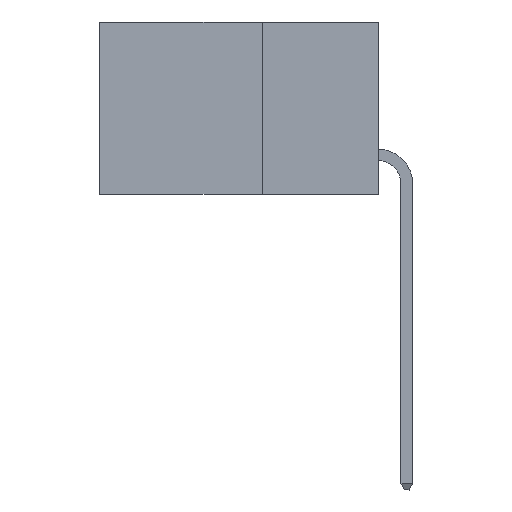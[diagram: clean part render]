
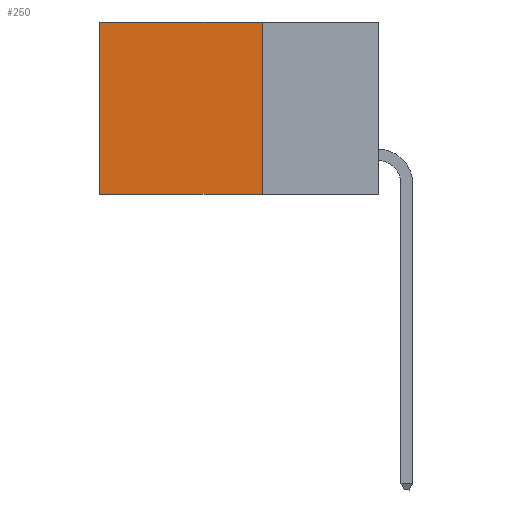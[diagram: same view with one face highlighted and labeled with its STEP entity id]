
A CAD part, left-side view. The second image highlights one B-rep face of the part: STEP entity #250.
In plain terms, the highlighted planar face has unit normal (-1, 0, 0).
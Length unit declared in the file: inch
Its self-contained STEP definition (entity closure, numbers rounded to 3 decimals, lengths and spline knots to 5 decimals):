
#130 = ORIENTED_EDGE ( 'NONE', *, *, #15612, .F. ) ;
#187 = CARTESIAN_POINT ( 'NONE',  ( 0.2615, 0.6, -0.37 ) ) ;
#250 = ADVANCED_FACE ( 'NONE', ( #16283 ), #5574, .F. ) ;
#1062 = LINE ( 'NONE', #5492, #11405 ) ;
#2078 = DIRECTION ( 'NONE',  ( 0., 0., -1. ) ) ;
#2416 = DIRECTION ( 'NONE',  ( 1., 0., 0. ) ) ;
#2471 = CARTESIAN_POINT ( 'NONE',  ( 0.2615, 0.25, -0.37 ) ) ;
#2823 = VECTOR ( 'NONE', #10074, 39.37008 ) ;
#4097 = AXIS2_PLACEMENT_3D ( 'NONE', #14981, #2416, #13232 ) ;
#4215 = DIRECTION ( 'NONE',  ( 0., 1., 0. ) ) ;
#4545 = EDGE_CURVE ( 'NONE', #11770, #15387, #1062, .T. ) ;
#5492 = CARTESIAN_POINT ( 'NONE',  ( 0.2615, 0.25, -0.37 ) ) ;
#5574 = PLANE ( 'NONE',  #4097 ) ;
#6549 = LINE ( 'NONE', #8162, #16066 ) ;
#6898 = CARTESIAN_POINT ( 'NONE',  ( 0.2615, 0.6, 0. ) ) ;
#7111 = ORIENTED_EDGE ( 'NONE', *, *, #4545, .F. ) ;
#8162 = CARTESIAN_POINT ( 'NONE',  ( 0.2615, 0.25, -0.37 ) ) ;
#9219 = VECTOR ( 'NONE', #4215, 39.37008 ) ;
#9790 = VERTEX_POINT ( 'NONE', #11768 ) ;
#10074 = DIRECTION ( 'NONE',  ( 0., 0., -1. ) ) ;
#10088 = DIRECTION ( 'NONE',  ( 0., 1., 0. ) ) ;
#11405 = VECTOR ( 'NONE', #10088, 39.37008 ) ;
#11606 = CARTESIAN_POINT ( 'NONE',  ( 0.2615, 0.6, -0.37 ) ) ;
#11768 = CARTESIAN_POINT ( 'NONE',  ( 0.2615, 0.25, 0. ) ) ;
#11770 = VERTEX_POINT ( 'NONE', #2471 ) ;
#13232 = DIRECTION ( 'NONE',  ( 0., 0., -1. ) ) ;
#14245 = LINE ( 'NONE', #11606, #2823 ) ;
#14891 = EDGE_CURVE ( 'NONE', #9790, #16611, #15317, .T. ) ;
#14937 = ORIENTED_EDGE ( 'NONE', *, *, #15170, .T. ) ;
#14981 = CARTESIAN_POINT ( 'NONE',  ( 0.2615, 0.25, -0.37 ) ) ;
#15170 = EDGE_CURVE ( 'NONE', #16611, #15387, #14245, .T. ) ;
#15317 = LINE ( 'NONE', #16627, #9219 ) ;
#15387 = VERTEX_POINT ( 'NONE', #187 ) ;
#15612 = EDGE_CURVE ( 'NONE', #9790, #11770, #6549, .T. ) ;
#16066 = VECTOR ( 'NONE', #2078, 39.37008 ) ;
#16283 = FACE_OUTER_BOUND ( 'NONE', #17725, .T. ) ;
#16611 = VERTEX_POINT ( 'NONE', #6898 ) ;
#16627 = CARTESIAN_POINT ( 'NONE',  ( 0.2615, 0.25, 0. ) ) ;
#17725 = EDGE_LOOP ( 'NONE', ( #14937, #7111, #130, #18288 ) ) ;
#18288 = ORIENTED_EDGE ( 'NONE', *, *, #14891, .T. ) ;
